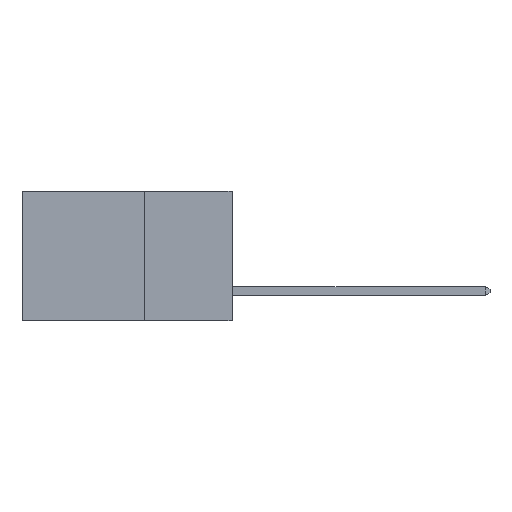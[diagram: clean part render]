
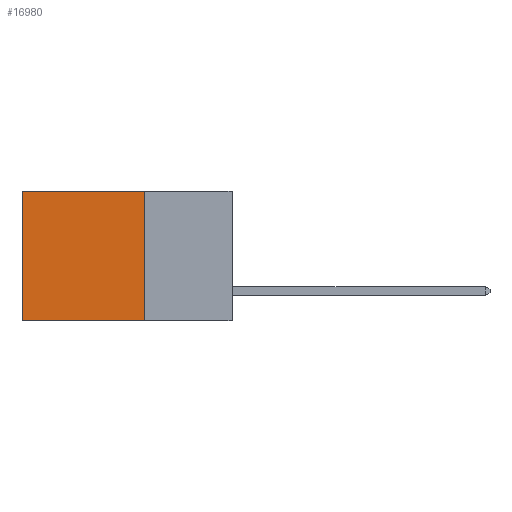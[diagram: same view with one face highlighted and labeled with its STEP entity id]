
A CAD part, left-side view. The second image highlights one B-rep face of the part: STEP entity #16980.
In plain terms, the highlighted planar face has unit normal (-1, 0, 0).
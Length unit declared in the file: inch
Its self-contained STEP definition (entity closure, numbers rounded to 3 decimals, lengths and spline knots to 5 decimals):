
#576 = CARTESIAN_POINT ( 'NONE',  ( 0.2875, 0.25, -0.37 ) ) ;
#642 = FACE_OUTER_BOUND ( 'NONE', #10535, .T. ) ;
#729 = VECTOR ( 'NONE', #4641, 39.37008 ) ;
#796 = CARTESIAN_POINT ( 'NONE',  ( 0.2875, 0.25, 0. ) ) ;
#2450 = DIRECTION ( 'NONE',  ( 1., 0., 0. ) ) ;
#3131 = VERTEX_POINT ( 'NONE', #5727 ) ;
#3558 = EDGE_CURVE ( 'NONE', #5020, #14129, #9316, .T. ) ;
#4023 = PLANE ( 'NONE',  #17963 ) ;
#4077 = LINE ( 'NONE', #7892, #7865 ) ;
#4641 = DIRECTION ( 'NONE',  ( 0., 0., -1. ) ) ;
#5013 = ORIENTED_EDGE ( 'NONE', *, *, #13411, .T. ) ;
#5020 = VERTEX_POINT ( 'NONE', #6340 ) ;
#5539 = ORIENTED_EDGE ( 'NONE', *, *, #3558, .F. ) ;
#5727 = CARTESIAN_POINT ( 'NONE',  ( 0.2875, 0.6, 0. ) ) ;
#6340 = CARTESIAN_POINT ( 'NONE',  ( 0.2875, 0.25, 0. ) ) ;
#7385 = ORIENTED_EDGE ( 'NONE', *, *, #15687, .T. ) ;
#7865 = VECTOR ( 'NONE', #10974, 39.37008 ) ;
#7892 = CARTESIAN_POINT ( 'NONE',  ( 0.2875, 0.6, 0. ) ) ;
#9316 = LINE ( 'NONE', #15640, #729 ) ;
#9782 = LINE ( 'NONE', #576, #13236 ) ;
#10251 = CARTESIAN_POINT ( 'NONE',  ( 0.2875, 0.25, 0. ) ) ;
#10535 = EDGE_LOOP ( 'NONE', ( #5013, #11215, #5539, #7385 ) ) ;
#10762 = VERTEX_POINT ( 'NONE', #17384 ) ;
#10779 = EDGE_CURVE ( 'NONE', #14129, #10762, #9782, .T. ) ;
#10974 = DIRECTION ( 'NONE',  ( 0., 0., -1. ) ) ;
#11215 = ORIENTED_EDGE ( 'NONE', *, *, #10779, .F. ) ;
#11729 = DIRECTION ( 'NONE',  ( 0., 1., 0. ) ) ;
#12714 = VECTOR ( 'NONE', #11729, 39.37008 ) ;
#12737 = CARTESIAN_POINT ( 'NONE',  ( 0.2875, 0.25, -0.37 ) ) ;
#13155 = LINE ( 'NONE', #10251, #12714 ) ;
#13236 = VECTOR ( 'NONE', #17448, 39.37008 ) ;
#13336 = DIRECTION ( 'NONE',  ( 0., 0., -1. ) ) ;
#13411 = EDGE_CURVE ( 'NONE', #3131, #10762, #4077, .T. ) ;
#14129 = VERTEX_POINT ( 'NONE', #12737 ) ;
#15640 = CARTESIAN_POINT ( 'NONE',  ( 0.2875, 0.25, 0. ) ) ;
#15687 = EDGE_CURVE ( 'NONE', #5020, #3131, #13155, .T. ) ;
#16980 = ADVANCED_FACE ( 'NONE', ( #642 ), #4023, .F. ) ;
#17384 = CARTESIAN_POINT ( 'NONE',  ( 0.2875, 0.6, -0.37 ) ) ;
#17448 = DIRECTION ( 'NONE',  ( 0., 1., 0. ) ) ;
#17963 = AXIS2_PLACEMENT_3D ( 'NONE', #796, #2450, #13336 ) ;
